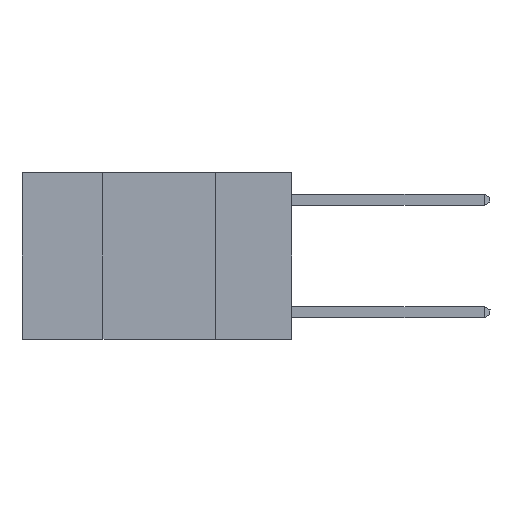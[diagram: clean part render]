
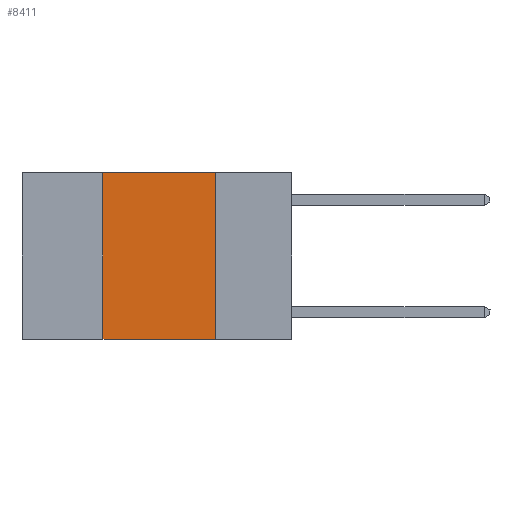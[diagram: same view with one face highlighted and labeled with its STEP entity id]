
A CAD part, left-side view. The second image highlights one B-rep face of the part: STEP entity #8411.
In plain terms, the highlighted planar face has unit normal (-1, 0, 0).
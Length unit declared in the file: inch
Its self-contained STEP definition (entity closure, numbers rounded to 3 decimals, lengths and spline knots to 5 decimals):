
#88 = PLANE ( 'NONE',  #3377 ) ;
#195 = VERTEX_POINT ( 'NONE', #12104 ) ;
#216 = ORIENTED_EDGE ( 'NONE', *, *, #8736, .F. ) ;
#248 = CARTESIAN_POINT ( 'NONE',  ( 0., 0.42, 0. ) ) ;
#671 = DIRECTION ( 'NONE',  ( 0., 0., 1. ) ) ;
#719 = CARTESIAN_POINT ( 'NONE',  ( 0., 0.17, 0. ) ) ;
#1292 = CARTESIAN_POINT ( 'NONE',  ( 0., 0.6, 0. ) ) ;
#1893 = EDGE_CURVE ( 'NONE', #5491, #5733, #12897, .T. ) ;
#1899 = LINE ( 'NONE', #14301, #7848 ) ;
#2578 = DIRECTION ( 'NONE',  ( 0., 0., -1. ) ) ;
#2720 = ORIENTED_EDGE ( 'NONE', *, *, #12438, .F. ) ;
#2745 = DIRECTION ( 'NONE',  ( 0., 0., -1. ) ) ;
#3377 = AXIS2_PLACEMENT_3D ( 'NONE', #1292, #9530, #2578 ) ;
#3756 = DIRECTION ( 'NONE',  ( 0., -1., 0. ) ) ;
#4455 = LINE ( 'NONE', #9480, #12677 ) ;
#4578 = CARTESIAN_POINT ( 'NONE',  ( 0., 0.6, 0. ) ) ;
#4622 = ORIENTED_EDGE ( 'NONE', *, *, #13954, .T. ) ;
#5206 = CARTESIAN_POINT ( 'NONE',  ( 0., 0.42, -0.37 ) ) ;
#5491 = VERTEX_POINT ( 'NONE', #248 ) ;
#5733 = VERTEX_POINT ( 'NONE', #719 ) ;
#6482 = LINE ( 'NONE', #9673, #12361 ) ;
#6925 = DIRECTION ( 'NONE',  ( 0., -1., 0. ) ) ;
#7848 = VECTOR ( 'NONE', #671, 39.37008 ) ;
#8411 = ADVANCED_FACE ( 'NONE', ( #11164 ), #88, .F. ) ;
#8736 = EDGE_CURVE ( 'NONE', #14121, #5491, #1899, .T. ) ;
#9480 = CARTESIAN_POINT ( 'NONE',  ( 0., 0.6, -0.37 ) ) ;
#9530 = DIRECTION ( 'NONE',  ( 1., 0., 0. ) ) ;
#9673 = CARTESIAN_POINT ( 'NONE',  ( 0., 0.17, 0. ) ) ;
#9988 = VECTOR ( 'NONE', #6925, 39.37008 ) ;
#11164 = FACE_OUTER_BOUND ( 'NONE', #12171, .T. ) ;
#12104 = CARTESIAN_POINT ( 'NONE',  ( 0., 0.17, -0.37 ) ) ;
#12171 = EDGE_LOOP ( 'NONE', ( #2720, #14649, #216, #4622 ) ) ;
#12361 = VECTOR ( 'NONE', #2745, 39.37008 ) ;
#12438 = EDGE_CURVE ( 'NONE', #5733, #195, #6482, .T. ) ;
#12677 = VECTOR ( 'NONE', #3756, 39.37008 ) ;
#12897 = LINE ( 'NONE', #4578, #9988 ) ;
#13954 = EDGE_CURVE ( 'NONE', #14121, #195, #4455, .T. ) ;
#14121 = VERTEX_POINT ( 'NONE', #5206 ) ;
#14301 = CARTESIAN_POINT ( 'NONE',  ( 0., 0.42, 0. ) ) ;
#14649 = ORIENTED_EDGE ( 'NONE', *, *, #1893, .F. ) ;
